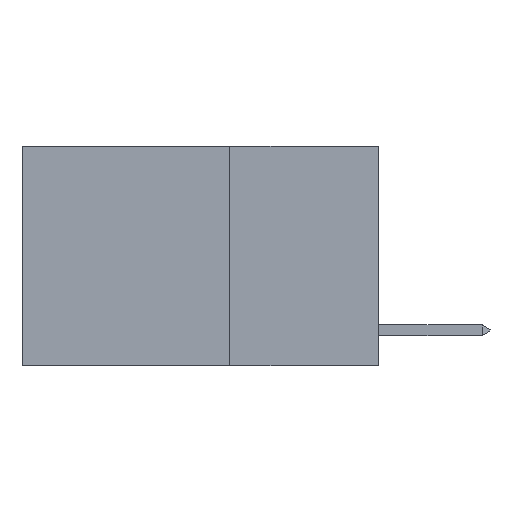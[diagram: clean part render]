
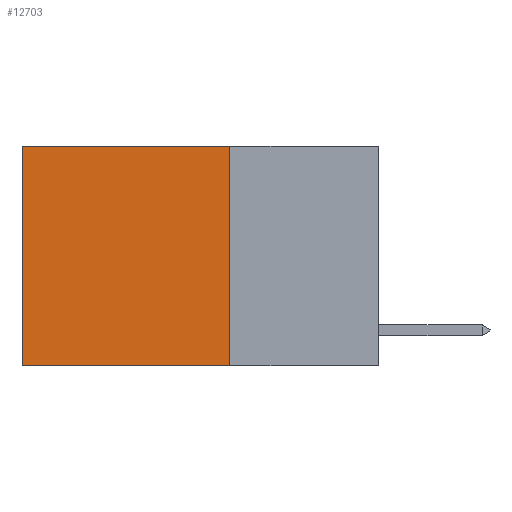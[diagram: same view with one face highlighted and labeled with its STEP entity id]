
A CAD part, left-side view. The second image highlights one B-rep face of the part: STEP entity #12703.
In plain terms, the highlighted planar face has unit normal (-1, 0, 0).
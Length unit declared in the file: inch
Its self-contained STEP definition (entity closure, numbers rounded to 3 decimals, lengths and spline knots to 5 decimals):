
#125 = EDGE_CURVE ( 'NONE', #20082, #13462, #16951, .T. ) ;
#287 = CARTESIAN_POINT ( 'NONE',  ( 0.2625, 0.25, 0. ) ) ;
#721 = CARTESIAN_POINT ( 'NONE',  ( 0.2625, 0.6, 0. ) ) ;
#741 = CARTESIAN_POINT ( 'NONE',  ( 0.2625, 0.25, -0.37 ) ) ;
#1656 = CARTESIAN_POINT ( 'NONE',  ( 0.2625, 0.25, 0. ) ) ;
#2695 = EDGE_LOOP ( 'NONE', ( #10094, #15728, #17664, #17330 ) ) ;
#3177 = CARTESIAN_POINT ( 'NONE',  ( 0.2625, 0.6, -0.37 ) ) ;
#4375 = DIRECTION ( 'NONE',  ( 0., 1., 0. ) ) ;
#5314 = LINE ( 'NONE', #741, #15657 ) ;
#5442 = VERTEX_POINT ( 'NONE', #17311 ) ;
#6103 = FACE_OUTER_BOUND ( 'NONE', #2695, .T. ) ;
#6937 = EDGE_CURVE ( 'NONE', #20082, #5442, #14948, .T. ) ;
#7757 = VECTOR ( 'NONE', #18844, 39.37008 ) ;
#8330 = LINE ( 'NONE', #721, #7757 ) ;
#10094 = ORIENTED_EDGE ( 'NONE', *, *, #17558, .T. ) ;
#10118 = VECTOR ( 'NONE', #21692, 39.37008 ) ;
#10921 = CARTESIAN_POINT ( 'NONE',  ( 0.2625, 0.25, 0. ) ) ;
#11219 = DIRECTION ( 'NONE',  ( 0., 0., -1. ) ) ;
#11234 = EDGE_CURVE ( 'NONE', #13462, #19073, #5314, .T. ) ;
#12093 = VECTOR ( 'NONE', #14510, 39.37008 ) ;
#12703 = ADVANCED_FACE ( 'NONE', ( #6103 ), #18475, .F. ) ;
#13462 = VERTEX_POINT ( 'NONE', #22405 ) ;
#14510 = DIRECTION ( 'NONE',  ( 0., 0., -1. ) ) ;
#14948 = LINE ( 'NONE', #1656, #10118 ) ;
#15171 = AXIS2_PLACEMENT_3D ( 'NONE', #287, #22113, #11219 ) ;
#15657 = VECTOR ( 'NONE', #4375, 39.37008 ) ;
#15728 = ORIENTED_EDGE ( 'NONE', *, *, #11234, .F. ) ;
#16951 = LINE ( 'NONE', #10921, #12093 ) ;
#17311 = CARTESIAN_POINT ( 'NONE',  ( 0.2625, 0.6, 0. ) ) ;
#17330 = ORIENTED_EDGE ( 'NONE', *, *, #6937, .T. ) ;
#17558 = EDGE_CURVE ( 'NONE', #5442, #19073, #8330, .T. ) ;
#17664 = ORIENTED_EDGE ( 'NONE', *, *, #125, .F. ) ;
#18475 = PLANE ( 'NONE',  #15171 ) ;
#18844 = DIRECTION ( 'NONE',  ( 0., 0., -1. ) ) ;
#19073 = VERTEX_POINT ( 'NONE', #3177 ) ;
#20082 = VERTEX_POINT ( 'NONE', #22612 ) ;
#21692 = DIRECTION ( 'NONE',  ( 0., 1., 0. ) ) ;
#22113 = DIRECTION ( 'NONE',  ( 1., 0., 0. ) ) ;
#22405 = CARTESIAN_POINT ( 'NONE',  ( 0.2625, 0.25, -0.37 ) ) ;
#22612 = CARTESIAN_POINT ( 'NONE',  ( 0.2625, 0.25, 0. ) ) ;
